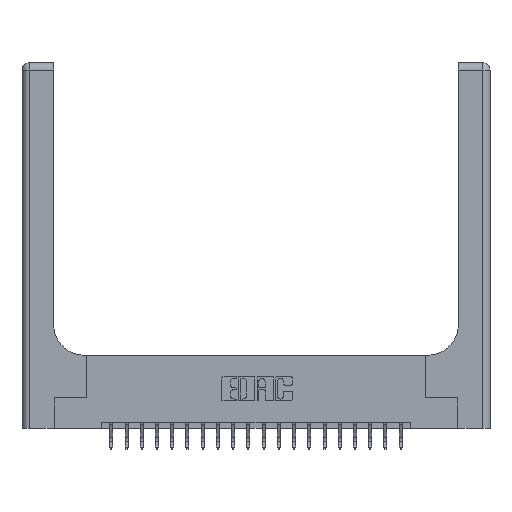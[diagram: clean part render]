
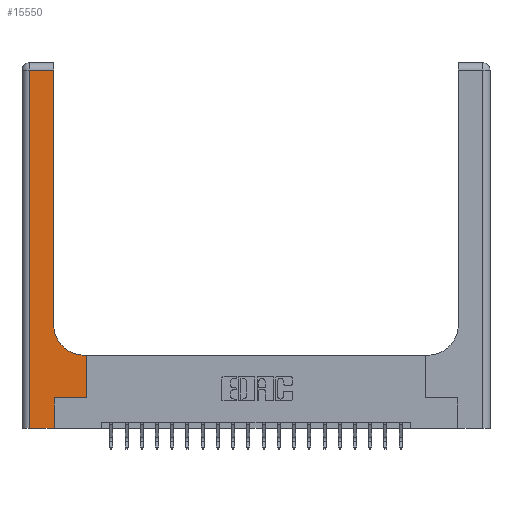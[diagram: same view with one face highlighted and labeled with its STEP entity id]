
A CAD part, top view. The second image highlights one B-rep face of the part: STEP entity #15550.
In plain terms, the highlighted planar face has unit normal (0, 0, 1).
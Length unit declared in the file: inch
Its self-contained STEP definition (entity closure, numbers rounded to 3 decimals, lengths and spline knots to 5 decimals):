
#2 = CARTESIAN_POINT ( 'NONE',  ( 0.26, 3., 0.37 ) ) ;
#44 = ORIENTED_EDGE ( 'NONE', *, *, #7325, .T. ) ;
#63 = EDGE_CURVE ( 'NONE', #6341, #20920, #19379, .T. ) ;
#441 = CARTESIAN_POINT ( 'NONE',  ( 0.265, 0., 0.37 ) ) ;
#545 = CARTESIAN_POINT ( 'NONE',  ( 0.528, 0.6, 0.37 ) ) ;
#1084 = VECTOR ( 'NONE', #17978, 39.37008 ) ;
#1905 = EDGE_CURVE ( 'NONE', #10287, #21151, #4794, .T. ) ;
#1962 = ORIENTED_EDGE ( 'NONE', *, *, #1905, .T. ) ;
#2235 = LINE ( 'NONE', #441, #5042 ) ;
#2267 = CARTESIAN_POINT ( 'NONE',  ( 0.51, 0.85, 0.37 ) ) ;
#2789 = CARTESIAN_POINT ( 'NONE',  ( 0.26, 0.85, 0.37 ) ) ;
#3226 = EDGE_CURVE ( 'NONE', #20920, #19472, #5502, .T. ) ;
#3356 = ORIENTED_EDGE ( 'NONE', *, *, #8923, .T. ) ;
#3524 = CARTESIAN_POINT ( 'NONE',  ( 0.26, 2.94, 0.37 ) ) ;
#4392 = LINE ( 'NONE', #4839, #4645 ) ;
#4645 = VECTOR ( 'NONE', #11498, 39.37008 ) ;
#4794 = CIRCLE ( 'NONE', #20449, 0.25 ) ;
#4839 = CARTESIAN_POINT ( 'NONE',  ( 0.528, 0.25, 0.37 ) ) ;
#5002 = DIRECTION ( 'NONE',  ( 1., 0., 0. ) ) ;
#5042 = VECTOR ( 'NONE', #11974, 39.37008 ) ;
#5313 = CARTESIAN_POINT ( 'NONE',  ( 0.06, 2.94, 0.37 ) ) ;
#5502 = LINE ( 'NONE', #12850, #16153 ) ;
#5953 = EDGE_CURVE ( 'NONE', #21151, #6341, #13969, .T. ) ;
#6341 = VERTEX_POINT ( 'NONE', #3524 ) ;
#6429 = ORIENTED_EDGE ( 'NONE', *, *, #63, .T. ) ;
#6999 = LINE ( 'NONE', #14680, #1084 ) ;
#7325 = EDGE_CURVE ( 'NONE', #19472, #11643, #8996, .T. ) ;
#7788 = CARTESIAN_POINT ( 'NONE',  ( 0., 3., 0.37 ) ) ;
#7859 = DIRECTION ( 'NONE',  ( -1., 0., 0. ) ) ;
#8215 = CARTESIAN_POINT ( 'NONE',  ( 0.528, 0.25, 0.37 ) ) ;
#8394 = ORIENTED_EDGE ( 'NONE', *, *, #18337, .T. ) ;
#8923 = EDGE_CURVE ( 'NONE', #11643, #21196, #2235, .T. ) ;
#8996 = LINE ( 'NONE', #21337, #14982 ) ;
#9938 = CARTESIAN_POINT ( 'NONE',  ( 0.06, 0., 0.37 ) ) ;
#10287 = VERTEX_POINT ( 'NONE', #11458 ) ;
#11124 = CARTESIAN_POINT ( 'NONE',  ( 0., 2.94, 0.37 ) ) ;
#11339 = DIRECTION ( 'NONE',  ( -1., 0., 0. ) ) ;
#11458 = CARTESIAN_POINT ( 'NONE',  ( 0.51, 0.6, 0.37 ) ) ;
#11484 = EDGE_CURVE ( 'NONE', #13001, #10287, #6999, .T. ) ;
#11498 = DIRECTION ( 'NONE',  ( 0., 1., 0. ) ) ;
#11624 = VECTOR ( 'NONE', #11711, 39.37008 ) ;
#11643 = VERTEX_POINT ( 'NONE', #14964 ) ;
#11711 = DIRECTION ( 'NONE',  ( 1., 0., 0. ) ) ;
#11786 = FACE_OUTER_BOUND ( 'NONE', #12045, .T. ) ;
#11974 = DIRECTION ( 'NONE',  ( 0., 1., 0. ) ) ;
#12045 = EDGE_LOOP ( 'NONE', ( #21380, #6429, #19426, #44, #3356, #8394, #12333, #19335, #1962 ) ) ;
#12073 = DIRECTION ( 'NONE',  ( 0., 0., -1. ) ) ;
#12333 = ORIENTED_EDGE ( 'NONE', *, *, #12900, .T. ) ;
#12779 = DIRECTION ( 'NONE',  ( 0., -1., 0. ) ) ;
#12846 = CARTESIAN_POINT ( 'NONE',  ( 0.265, 0.25, 0.37 ) ) ;
#12850 = CARTESIAN_POINT ( 'NONE',  ( 0.06, 3., 0.37 ) ) ;
#12900 = EDGE_CURVE ( 'NONE', #17497, #13001, #4392, .T. ) ;
#13001 = VERTEX_POINT ( 'NONE', #545 ) ;
#13488 = DIRECTION ( 'NONE',  ( 0., 1., 0. ) ) ;
#13969 = LINE ( 'NONE', #2, #21249 ) ;
#14216 = AXIS2_PLACEMENT_3D ( 'NONE', #7788, #15921, #7859 ) ;
#14311 = PLANE ( 'NONE',  #14216 ) ;
#14680 = CARTESIAN_POINT ( 'NONE',  ( 0.26, 0.6, 0.37 ) ) ;
#14964 = CARTESIAN_POINT ( 'NONE',  ( 0.265, 0., 0.37 ) ) ;
#14982 = VECTOR ( 'NONE', #5002, 39.37008 ) ;
#15423 = DIRECTION ( 'NONE',  ( 1., 0., 0. ) ) ;
#15550 = ADVANCED_FACE ( 'NONE', ( #11786 ), #14311, .F. ) ;
#15921 = DIRECTION ( 'NONE',  ( 0., 0., -1. ) ) ;
#16053 = LINE ( 'NONE', #16742, #11624 ) ;
#16153 = VECTOR ( 'NONE', #12779, 39.37008 ) ;
#16742 = CARTESIAN_POINT ( 'NONE',  ( 0.265, 0.25, 0.37 ) ) ;
#17497 = VERTEX_POINT ( 'NONE', #8215 ) ;
#17978 = DIRECTION ( 'NONE',  ( -1., 0., 0. ) ) ;
#18337 = EDGE_CURVE ( 'NONE', #21196, #17497, #16053, .T. ) ;
#18877 = VECTOR ( 'NONE', #11339, 39.37008 ) ;
#19335 = ORIENTED_EDGE ( 'NONE', *, *, #11484, .T. ) ;
#19379 = LINE ( 'NONE', #11124, #18877 ) ;
#19426 = ORIENTED_EDGE ( 'NONE', *, *, #3226, .T. ) ;
#19472 = VERTEX_POINT ( 'NONE', #9938 ) ;
#20449 = AXIS2_PLACEMENT_3D ( 'NONE', #2267, #12073, #15423 ) ;
#20920 = VERTEX_POINT ( 'NONE', #5313 ) ;
#21151 = VERTEX_POINT ( 'NONE', #2789 ) ;
#21196 = VERTEX_POINT ( 'NONE', #12846 ) ;
#21249 = VECTOR ( 'NONE', #13488, 39.37008 ) ;
#21337 = CARTESIAN_POINT ( 'NONE',  ( 0., 0., 0.37 ) ) ;
#21380 = ORIENTED_EDGE ( 'NONE', *, *, #5953, .T. ) ;
